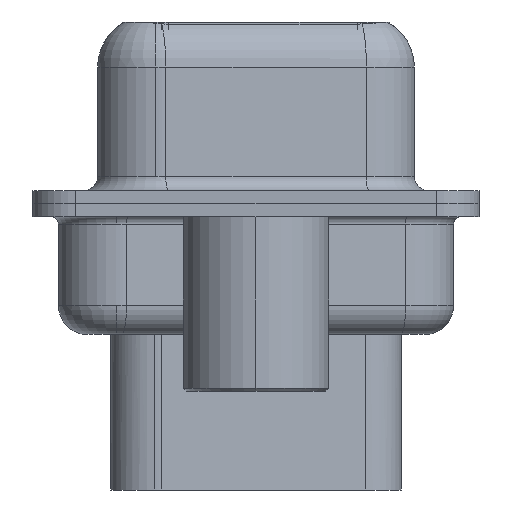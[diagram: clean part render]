
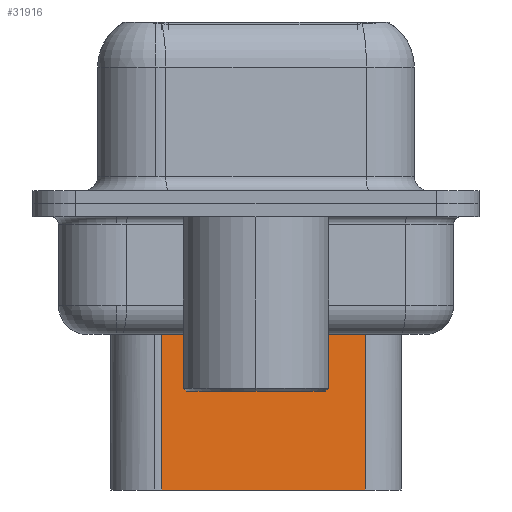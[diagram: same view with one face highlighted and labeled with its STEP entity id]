
A CAD part, left-side view. The second image highlights one B-rep face of the part: STEP entity #31916.
In plain terms, the highlighted planar face has unit normal (-0.985, -0.174, 0).
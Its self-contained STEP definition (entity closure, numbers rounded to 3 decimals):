
#1549 = DIRECTION ( 'NONE',  ( 0.174, -0.985, 0. ) ) ;
#2868 = DIRECTION ( 'NONE',  ( 0., 0., -1. ) ) ;
#3416 = EDGE_CURVE ( 'NONE', #32535, #18816, #34470, .T. ) ;
#4265 = VECTOR ( 'NONE', #4991, 1000. ) ;
#4991 = DIRECTION ( 'NONE',  ( -0.174, 0.985, 0. ) ) ;
#5021 = DIRECTION ( 'NONE',  ( -0.174, 0.985, 0. ) ) ;
#5412 = CARTESIAN_POINT ( 'NONE',  ( 5.858, -3.76, -9.85 ) ) ;
#5493 = CARTESIAN_POINT ( 'NONE',  ( 4.624, 3.24, -3.975 ) ) ;
#6581 = VERTEX_POINT ( 'NONE', #27382 ) ;
#7205 = EDGE_LOOP ( 'NONE', ( #35551, #23654, #30101, #23412 ) ) ;
#7956 = CARTESIAN_POINT ( 'NONE',  ( 4.624, 3.24, -9.85 ) ) ;
#8102 = CARTESIAN_POINT ( 'NONE',  ( 4.453, 4.209, -3.975 ) ) ;
#8142 = EDGE_CURVE ( 'NONE', #20328, #18816, #35453, .T. ) ;
#8382 = DIRECTION ( 'NONE',  ( 0., 0., -1. ) ) ;
#18816 = VERTEX_POINT ( 'NONE', #37666 ) ;
#19546 = DIRECTION ( 'NONE',  ( -0.985, -0.174, 0. ) ) ;
#20328 = VERTEX_POINT ( 'NONE', #5493 ) ;
#20375 = CARTESIAN_POINT ( 'NONE',  ( 4.624, 3.24, -3.1 ) ) ;
#20471 = VECTOR ( 'NONE', #2868, 1000. ) ;
#20492 = LINE ( 'NONE', #29784, #20471 ) ;
#20715 = VECTOR ( 'NONE', #8382, 1000. ) ;
#23412 = ORIENTED_EDGE ( 'NONE', *, *, #3416, .F. ) ;
#23654 = ORIENTED_EDGE ( 'NONE', *, *, #25556, .T. ) ;
#24787 = FACE_OUTER_BOUND ( 'NONE', #7205, .T. ) ;
#25162 = VECTOR ( 'NONE', #5021, 1000. ) ;
#25556 = EDGE_CURVE ( 'NONE', #6581, #20328, #28257, .T. ) ;
#26904 = AXIS2_PLACEMENT_3D ( 'NONE', #33882, #19546, #1549 ) ;
#27015 = EDGE_CURVE ( 'NONE', #6581, #32535, #20492, .T. ) ;
#27382 = CARTESIAN_POINT ( 'NONE',  ( 5.858, -3.76, -3.975 ) ) ;
#28257 = LINE ( 'NONE', #8102, #4265 ) ;
#29784 = CARTESIAN_POINT ( 'NONE',  ( 5.858, -3.76, -3.1 ) ) ;
#30101 = ORIENTED_EDGE ( 'NONE', *, *, #8142, .T. ) ;
#31916 = ADVANCED_FACE ( 'NONE', ( #24787 ), #33690, .T. ) ;
#32535 = VERTEX_POINT ( 'NONE', #5412 ) ;
#33690 = PLANE ( 'NONE',  #26904 ) ;
#33882 = CARTESIAN_POINT ( 'NONE',  ( 4.624, 3.24, -3.1 ) ) ;
#34470 = LINE ( 'NONE', #7956, #25162 ) ;
#35453 = LINE ( 'NONE', #20375, #20715 ) ;
#35551 = ORIENTED_EDGE ( 'NONE', *, *, #27015, .F. ) ;
#37666 = CARTESIAN_POINT ( 'NONE',  ( 4.624, 3.24, -9.85 ) ) ;
